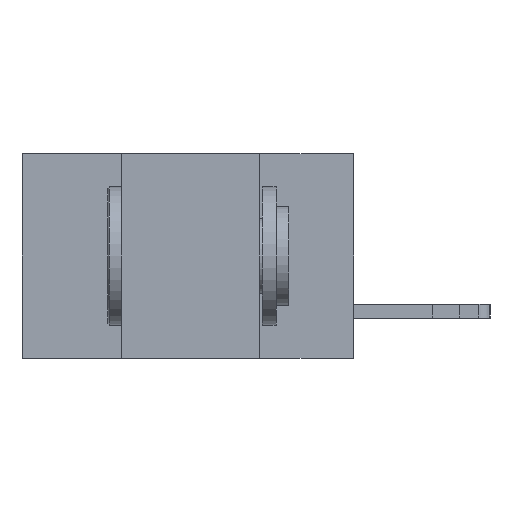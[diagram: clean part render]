
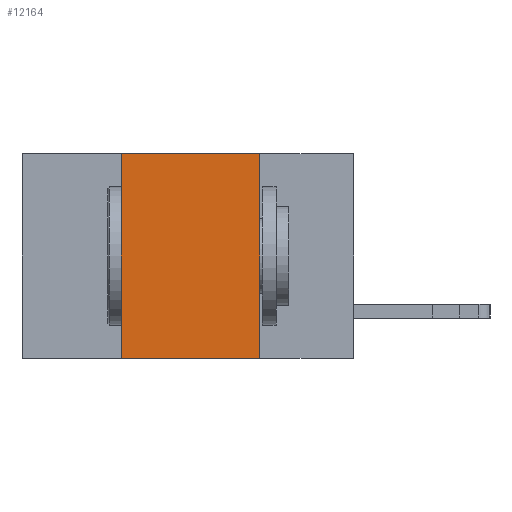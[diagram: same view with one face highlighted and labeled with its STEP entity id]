
A CAD part, left-side view. The second image highlights one B-rep face of the part: STEP entity #12164.
In plain terms, the highlighted planar face has unit normal (-1, 0, 0).
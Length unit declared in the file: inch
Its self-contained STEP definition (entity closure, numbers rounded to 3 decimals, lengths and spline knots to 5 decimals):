
#400 = DIRECTION ( 'NONE',  ( 1., 0., 0. ) ) ;
#556 = AXIS2_PLACEMENT_3D ( 'NONE', #14230, #400, #7953 ) ;
#799 = VECTOR ( 'NONE', #4635, 39.37008 ) ;
#1095 = LINE ( 'NONE', #6333, #11037 ) ;
#1297 = EDGE_LOOP ( 'NONE', ( #10544, #1473, #4228, #9284 ) ) ;
#1473 = ORIENTED_EDGE ( 'NONE', *, *, #11797, .F. ) ;
#2094 = CARTESIAN_POINT ( 'NONE',  ( 0., 0.42, -0.37 ) ) ;
#2409 = LINE ( 'NONE', #7420, #799 ) ;
#2699 = DIRECTION ( 'NONE',  ( 0., 0., -1. ) ) ;
#2765 = CARTESIAN_POINT ( 'NONE',  ( 0., 0.17, 0. ) ) ;
#3177 = VERTEX_POINT ( 'NONE', #15900 ) ;
#3564 = DIRECTION ( 'NONE',  ( 0., 0., 1. ) ) ;
#3717 = VECTOR ( 'NONE', #3564, 39.37008 ) ;
#4228 = ORIENTED_EDGE ( 'NONE', *, *, #16007, .F. ) ;
#4408 = VERTEX_POINT ( 'NONE', #11553 ) ;
#4635 = DIRECTION ( 'NONE',  ( 0., -1., 0. ) ) ;
#6333 = CARTESIAN_POINT ( 'NONE',  ( 0., 0.6, 0. ) ) ;
#7420 = CARTESIAN_POINT ( 'NONE',  ( 0., 0.6, -0.37 ) ) ;
#7519 = VERTEX_POINT ( 'NONE', #2094 ) ;
#7537 = CARTESIAN_POINT ( 'NONE',  ( 0., 0.17, 0. ) ) ;
#7953 = DIRECTION ( 'NONE',  ( 0., 0., -1. ) ) ;
#8490 = CARTESIAN_POINT ( 'NONE',  ( 0., 0.42, 0. ) ) ;
#9284 = ORIENTED_EDGE ( 'NONE', *, *, #16013, .T. ) ;
#10242 = PLANE ( 'NONE',  #556 ) ;
#10325 = FACE_OUTER_BOUND ( 'NONE', #1297, .T. ) ;
#10544 = ORIENTED_EDGE ( 'NONE', *, *, #12400, .F. ) ;
#11037 = VECTOR ( 'NONE', #11116, 39.37008 ) ;
#11116 = DIRECTION ( 'NONE',  ( 0., -1., 0. ) ) ;
#11553 = CARTESIAN_POINT ( 'NONE',  ( 0., 0.17, -0.37 ) ) ;
#11797 = EDGE_CURVE ( 'NONE', #3177, #14022, #1095, .T. ) ;
#12164 = ADVANCED_FACE ( 'NONE', ( #10325 ), #10242, .F. ) ;
#12400 = EDGE_CURVE ( 'NONE', #14022, #4408, #13829, .T. ) ;
#13829 = LINE ( 'NONE', #7537, #15795 ) ;
#14022 = VERTEX_POINT ( 'NONE', #2765 ) ;
#14230 = CARTESIAN_POINT ( 'NONE',  ( 0., 0.6, 0. ) ) ;
#14695 = LINE ( 'NONE', #8490, #3717 ) ;
#15795 = VECTOR ( 'NONE', #2699, 39.37008 ) ;
#15900 = CARTESIAN_POINT ( 'NONE',  ( 0., 0.42, 0. ) ) ;
#16007 = EDGE_CURVE ( 'NONE', #7519, #3177, #14695, .T. ) ;
#16013 = EDGE_CURVE ( 'NONE', #7519, #4408, #2409, .T. ) ;
